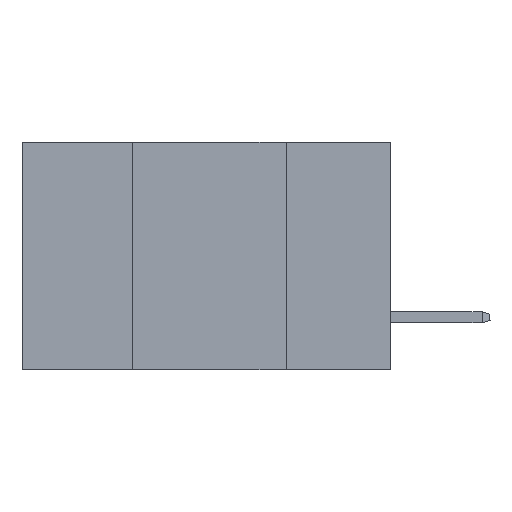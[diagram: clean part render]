
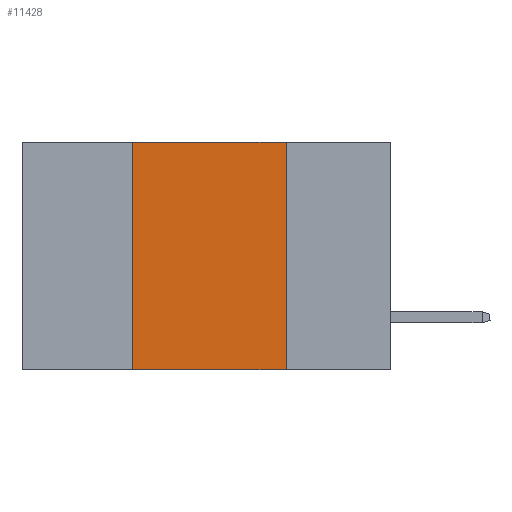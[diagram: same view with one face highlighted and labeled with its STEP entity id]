
A CAD part, left-side view. The second image highlights one B-rep face of the part: STEP entity #11428.
In plain terms, the highlighted planar face has unit normal (-1, 0, 0).
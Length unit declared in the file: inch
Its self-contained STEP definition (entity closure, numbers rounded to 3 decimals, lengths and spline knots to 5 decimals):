
#2421 = DIRECTION ( 'NONE',  ( 0., 0., 1. ) ) ;
#2752 = ORIENTED_EDGE ( 'NONE', *, *, #9719, .F. ) ;
#2914 = VERTEX_POINT ( 'NONE', #12184 ) ;
#3727 = VECTOR ( 'NONE', #13317, 39.37008 ) ;
#4906 = EDGE_LOOP ( 'NONE', ( #7777, #2752, #14058, #18029 ) ) ;
#5605 = CARTESIAN_POINT ( 'NONE',  ( 0., 0.42, 0. ) ) ;
#6033 = VECTOR ( 'NONE', #11403, 39.37008 ) ;
#7140 = LINE ( 'NONE', #10700, #11058 ) ;
#7270 = DIRECTION ( 'NONE',  ( 0., -1., 0. ) ) ;
#7316 = DIRECTION ( 'NONE',  ( 1., 0., 0. ) ) ;
#7389 = DIRECTION ( 'NONE',  ( 0., 0., -1. ) ) ;
#7777 = ORIENTED_EDGE ( 'NONE', *, *, #10751, .F. ) ;
#8200 = LINE ( 'NONE', #11521, #3727 ) ;
#9127 = VERTEX_POINT ( 'NONE', #12704 ) ;
#9719 = EDGE_CURVE ( 'NONE', #20418, #18467, #8200, .T. ) ;
#10131 = EDGE_CURVE ( 'NONE', #9127, #2914, #7140, .T. ) ;
#10700 = CARTESIAN_POINT ( 'NONE',  ( 0., 0.6, -0.37 ) ) ;
#10751 = EDGE_CURVE ( 'NONE', #18467, #2914, #15842, .T. ) ;
#11058 = VECTOR ( 'NONE', #7270, 39.37008 ) ;
#11403 = DIRECTION ( 'NONE',  ( 0., 0., -1. ) ) ;
#11428 = ADVANCED_FACE ( 'NONE', ( #16866 ), #17081, .F. ) ;
#11521 = CARTESIAN_POINT ( 'NONE',  ( 0., 0.6, 0. ) ) ;
#12184 = CARTESIAN_POINT ( 'NONE',  ( 0., 0.17, -0.37 ) ) ;
#12439 = EDGE_CURVE ( 'NONE', #9127, #20418, #16038, .T. ) ;
#12704 = CARTESIAN_POINT ( 'NONE',  ( 0., 0.42, -0.37 ) ) ;
#12844 = CARTESIAN_POINT ( 'NONE',  ( 0., 0.17, 0. ) ) ;
#13317 = DIRECTION ( 'NONE',  ( 0., -1., 0. ) ) ;
#14058 = ORIENTED_EDGE ( 'NONE', *, *, #12439, .F. ) ;
#15454 = CARTESIAN_POINT ( 'NONE',  ( 0., 0.6, 0. ) ) ;
#15842 = LINE ( 'NONE', #12844, #6033 ) ;
#16038 = LINE ( 'NONE', #5605, #19446 ) ;
#16866 = FACE_OUTER_BOUND ( 'NONE', #4906, .T. ) ;
#17081 = PLANE ( 'NONE',  #17160 ) ;
#17160 = AXIS2_PLACEMENT_3D ( 'NONE', #15454, #7316, #7389 ) ;
#18029 = ORIENTED_EDGE ( 'NONE', *, *, #10131, .T. ) ;
#18155 = CARTESIAN_POINT ( 'NONE',  ( 0., 0.17, 0. ) ) ;
#18467 = VERTEX_POINT ( 'NONE', #18155 ) ;
#18529 = CARTESIAN_POINT ( 'NONE',  ( 0., 0.42, 0. ) ) ;
#19446 = VECTOR ( 'NONE', #2421, 39.37008 ) ;
#20418 = VERTEX_POINT ( 'NONE', #18529 ) ;
